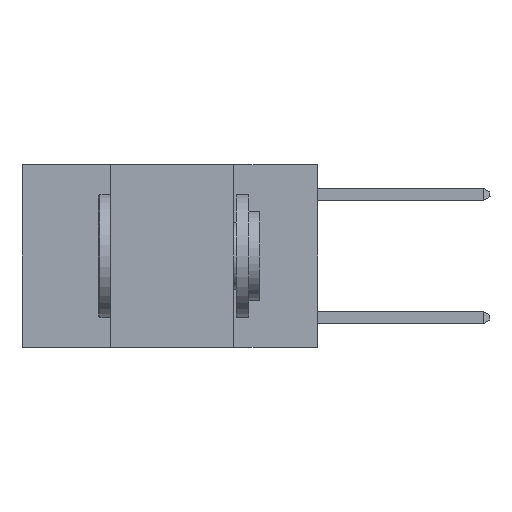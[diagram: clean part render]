
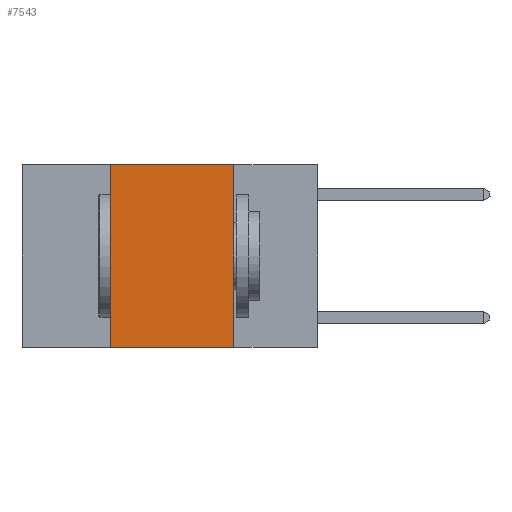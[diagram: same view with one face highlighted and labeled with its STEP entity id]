
A CAD part, left-side view. The second image highlights one B-rep face of the part: STEP entity #7543.
In plain terms, the highlighted planar face has unit normal (-1, 0, 0).
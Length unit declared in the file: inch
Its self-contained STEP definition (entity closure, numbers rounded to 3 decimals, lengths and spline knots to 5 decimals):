
#207 = ORIENTED_EDGE ( 'NONE', *, *, #3094, .F. ) ;
#643 = EDGE_CURVE ( 'NONE', #853, #6934, #10290, .T. ) ;
#853 = VERTEX_POINT ( 'NONE', #3208 ) ;
#871 = CARTESIAN_POINT ( 'NONE',  ( 0., 0.6, 0. ) ) ;
#1835 = DIRECTION ( 'NONE',  ( 0., 0., -1. ) ) ;
#2511 = EDGE_CURVE ( 'NONE', #853, #5834, #6295, .T. ) ;
#2679 = PLANE ( 'NONE',  #4582 ) ;
#2946 = ORIENTED_EDGE ( 'NONE', *, *, #11075, .F. ) ;
#3005 = VERTEX_POINT ( 'NONE', #4424 ) ;
#3029 = CARTESIAN_POINT ( 'NONE',  ( 0., 0.42, 0. ) ) ;
#3094 = EDGE_CURVE ( 'NONE', #3005, #6934, #4858, .T. ) ;
#3208 = CARTESIAN_POINT ( 'NONE',  ( 0., 0.42, -0.37 ) ) ;
#3471 = ORIENTED_EDGE ( 'NONE', *, *, #2511, .F. ) ;
#4424 = CARTESIAN_POINT ( 'NONE',  ( 0., 0.17, 0. ) ) ;
#4550 = VECTOR ( 'NONE', #9952, 39.37008 ) ;
#4582 = AXIS2_PLACEMENT_3D ( 'NONE', #871, #7270, #1835 ) ;
#4596 = DIRECTION ( 'NONE',  ( 0., -1., 0. ) ) ;
#4858 = LINE ( 'NONE', #6538, #4550 ) ;
#5182 = CARTESIAN_POINT ( 'NONE',  ( 0., 0.42, 0. ) ) ;
#5495 = VECTOR ( 'NONE', #4596, 39.37008 ) ;
#5778 = LINE ( 'NONE', #10645, #10286 ) ;
#5787 = DIRECTION ( 'NONE',  ( 0., 0., 1. ) ) ;
#5834 = VERTEX_POINT ( 'NONE', #5182 ) ;
#6294 = ORIENTED_EDGE ( 'NONE', *, *, #643, .T. ) ;
#6295 = LINE ( 'NONE', #3029, #11024 ) ;
#6538 = CARTESIAN_POINT ( 'NONE',  ( 0., 0.17, 0. ) ) ;
#6934 = VERTEX_POINT ( 'NONE', #10897 ) ;
#7270 = DIRECTION ( 'NONE',  ( 1., 0., 0. ) ) ;
#7543 = ADVANCED_FACE ( 'NONE', ( #7544 ), #2679, .F. ) ;
#7544 = FACE_OUTER_BOUND ( 'NONE', #8839, .T. ) ;
#7967 = DIRECTION ( 'NONE',  ( 0., -1., 0. ) ) ;
#8839 = EDGE_LOOP ( 'NONE', ( #207, #2946, #3471, #6294 ) ) ;
#9097 = CARTESIAN_POINT ( 'NONE',  ( 0., 0.6, -0.37 ) ) ;
#9952 = DIRECTION ( 'NONE',  ( 0., 0., -1. ) ) ;
#10286 = VECTOR ( 'NONE', #7967, 39.37008 ) ;
#10290 = LINE ( 'NONE', #9097, #5495 ) ;
#10645 = CARTESIAN_POINT ( 'NONE',  ( 0., 0.6, 0. ) ) ;
#10897 = CARTESIAN_POINT ( 'NONE',  ( 0., 0.17, -0.37 ) ) ;
#11024 = VECTOR ( 'NONE', #5787, 39.37008 ) ;
#11075 = EDGE_CURVE ( 'NONE', #5834, #3005, #5778, .T. ) ;
